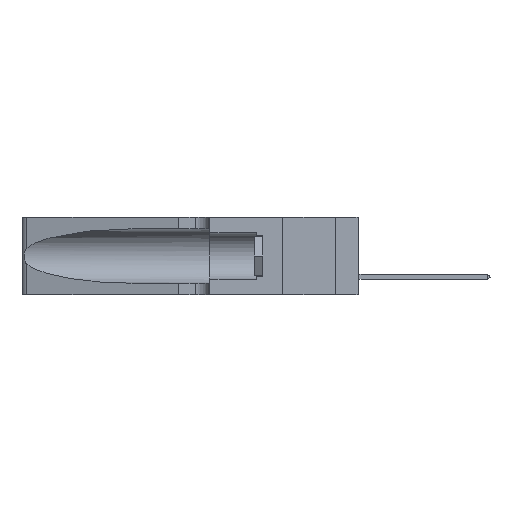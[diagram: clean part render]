
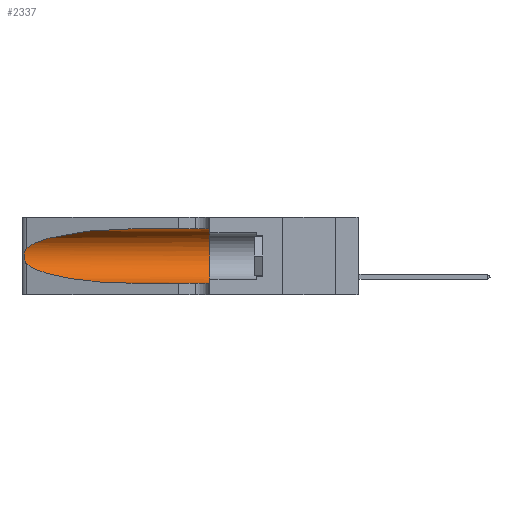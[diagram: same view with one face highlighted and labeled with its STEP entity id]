
A CAD part, left-side view. The second image highlights one B-rep face of the part: STEP entity #2337.
In plain terms, the highlighted cylindrical face has radius 3.308 mm (diameter 6.617 mm), a partial arc.
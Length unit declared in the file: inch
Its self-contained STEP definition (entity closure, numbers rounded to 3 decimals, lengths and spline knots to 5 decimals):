
#454 = CARTESIAN_POINT ( 'NONE',  ( 0.26075, 1.23896, 0.178 ) ) ;
#2295 = CARTESIAN_POINT ( 'NONE',  ( 0.25854, 1.2359, 0.20912 ) ) ;
#2337 = ADVANCED_FACE ( 'NONE', ( #6462 ), #10095, .F. ) ;
#2697 = EDGE_CURVE ( 'NONE', #14906, #32252, #18087, .T. ) ;
#2852 = VERTEX_POINT ( 'NONE', #28870 ) ;
#3932 = CARTESIAN_POINT ( 'NONE',  ( 0.1305, 0.72297, 0.31525 ) ) ;
#4654 = ORIENTED_EDGE ( 'NONE', *, *, #2697, .F. ) ;
#5775 = EDGE_CURVE ( 'NONE', #32252, #12425, #25843, .T. ) ;
#6020 = CARTESIAN_POINT ( 'NONE',  ( 0.2373, 1.15595, 0.08982 ) ) ;
#6446 = VERTEX_POINT ( 'NONE', #31807 ) ;
#6462 = FACE_OUTER_BOUND ( 'NONE', #29923, .T. ) ;
#6856 = VECTOR ( 'NONE', #22949, 39.37008 ) ;
#7241 = CARTESIAN_POINT ( 'NONE',  ( 0.25487, 1.22718, 0.22369 ) ) ;
#7370 = CARTESIAN_POINT ( 'NONE',  ( 0.25856, 1.23593, 0.16098 ) ) ;
#7404 = EDGE_CURVE ( 'NONE', #2852, #6446, #10278, .T. ) ;
#7745 = CARTESIAN_POINT ( 'NONE',  ( 0.1305, 1.61858, 0.31525 ) ) ;
#9529 = CARTESIAN_POINT ( 'NONE',  ( 0.1305, 0.72297, 0.05475 ) ) ;
#10095 = CYLINDRICAL_SURFACE ( 'NONE', #30429, 0.13025 ) ;
#10278 =( BOUNDED_CURVE ( )  B_SPLINE_CURVE ( 3, ( #33264, #6020, #31764, #9529 ),
 .UNSPECIFIED., .F., .T. ) 
 B_SPLINE_CURVE_WITH_KNOTS ( ( 4, 4 ),
 ( 3.44316, 4.71239 ),
 .UNSPECIFIED. ) 
 CURVE ( )  GEOMETRIC_REPRESENTATION_ITEM ( )  RATIONAL_B_SPLINE_CURVE ( ( 1., 0.87, 0.87, 1. ) ) 
 REPRESENTATION_ITEM ( '' )  );
#10597 = CARTESIAN_POINT ( 'NONE',  ( 0.26075, 1.23896, 0.19203 ) ) ;
#11135 = CARTESIAN_POINT ( 'NONE',  ( 0.1305, 1.61858, 0.185 ) ) ;
#11465 = DIRECTION ( 'NONE',  ( 0., 0., -1. ) ) ;
#11824 = DIRECTION ( 'NONE',  ( 0., 1., 0. ) ) ;
#12232 = CARTESIAN_POINT ( 'NONE',  ( 0.18966, 0.96281, 0.31525 ) ) ;
#12425 = VERTEX_POINT ( 'NONE', #19423 ) ;
#13458 = CARTESIAN_POINT ( 'NONE',  ( 0.1305, 1.61858, 0.05475 ) ) ;
#14906 = VERTEX_POINT ( 'NONE', #3932 ) ;
#15258 = CARTESIAN_POINT ( 'NONE',  ( 0.26018, 1.23835, 0.19895 ) ) ;
#15892 = CARTESIAN_POINT ( 'NONE',  ( 0.25789, 1.23486, 0.15765 ) ) ;
#15894 = EDGE_CURVE ( 'NONE', #6446, #12425, #19828, .T. ) ;
#17557 = AXIS2_PLACEMENT_3D ( 'NONE', #27231, #11824, #27682 ) ;
#17828 = CARTESIAN_POINT ( 'NONE',  ( 0.25555, 1.22993, 0.14849 ) ) ;
#18087 = LINE ( 'NONE', #7745, #6856 ) ;
#18279 =( BOUNDED_CURVE ( )  B_SPLINE_CURVE ( 3, ( #32993, #12232, #25368, #7241 ),
 .UNSPECIFIED., .F., .T. ) 
 B_SPLINE_CURVE_WITH_KNOTS ( ( 4, 4 ),
 ( 1.5708, 2.84003 ),
 .UNSPECIFIED. ) 
 CURVE ( )  GEOMETRIC_REPRESENTATION_ITEM ( )  RATIONAL_B_SPLINE_CURVE ( ( 1., 0.87, 0.87, 1. ) ) 
 REPRESENTATION_ITEM ( '' )  );
#18993 = VECTOR ( 'NONE', #31418, 39.37008 ) ;
#19423 = CARTESIAN_POINT ( 'NONE',  ( 0.1305, 0.35, 0.05475 ) ) ;
#19443 = ORIENTED_EDGE ( 'NONE', *, *, #5775, .F. ) ;
#19828 = LINE ( 'NONE', #13458, #18993 ) ;
#20319 = CARTESIAN_POINT ( 'NONE',  ( 0.25787, 1.23484, 0.2124 ) ) ;
#20538 = ORIENTED_EDGE ( 'NONE', *, *, #15894, .T. ) ;
#21029 = EDGE_CURVE ( 'NONE', #27607, #2852, #32774, .T. ) ;
#22562 = ORIENTED_EDGE ( 'NONE', *, *, #7404, .T. ) ;
#22949 = DIRECTION ( 'NONE',  ( 0., -1., 0. ) ) ;
#22960 = EDGE_CURVE ( 'NONE', #14906, #27607, #18279, .T. ) ;
#23156 = ORIENTED_EDGE ( 'NONE', *, *, #21029, .T. ) ;
#25368 = CARTESIAN_POINT ( 'NONE',  ( 0.2373, 1.15595, 0.28018 ) ) ;
#25386 = CARTESIAN_POINT ( 'NONE',  ( 0.25639, 1.23186, 0.15144 ) ) ;
#25495 = CARTESIAN_POINT ( 'NONE',  ( 0.25487, 1.22718, 0.22369 ) ) ;
#25510 = CARTESIAN_POINT ( 'NONE',  ( 0.25487, 1.22718, 0.22369 ) ) ;
#25843 = CIRCLE ( 'NONE', #17557, 0.13025 ) ;
#26920 = CARTESIAN_POINT ( 'NONE',  ( 0.1305, 0.35, 0.31525 ) ) ;
#27231 = CARTESIAN_POINT ( 'NONE',  ( 0.1305, 0.35, 0.185 ) ) ;
#27607 = VERTEX_POINT ( 'NONE', #25510 ) ;
#27682 = DIRECTION ( 'NONE',  ( 0., 0., 1. ) ) ;
#27969 = CARTESIAN_POINT ( 'NONE',  ( 0.26017, 1.23833, 0.17102 ) ) ;
#28849 = CARTESIAN_POINT ( 'NONE',  ( 0.25487, 1.22718, 0.14631 ) ) ;
#28870 = CARTESIAN_POINT ( 'NONE',  ( 0.25487, 1.22718, 0.14631 ) ) ;
#29145 = DIRECTION ( 'NONE',  ( 0., -1., 0. ) ) ;
#29923 = EDGE_LOOP ( 'NONE', ( #32422, #23156, #22562, #20538, #19443, #4654 ) ) ;
#30429 = AXIS2_PLACEMENT_3D ( 'NONE', #11135, #29145, #11465 ) ;
#30646 = CARTESIAN_POINT ( 'NONE',  ( 0.25639, 1.23184, 0.21858 ) ) ;
#31418 = DIRECTION ( 'NONE',  ( 0., -1., 0. ) ) ;
#31764 = CARTESIAN_POINT ( 'NONE',  ( 0.18966, 0.96281, 0.05475 ) ) ;
#31807 = CARTESIAN_POINT ( 'NONE',  ( 0.1305, 0.72297, 0.05475 ) ) ;
#32252 = VERTEX_POINT ( 'NONE', #26920 ) ;
#32422 = ORIENTED_EDGE ( 'NONE', *, *, #22960, .T. ) ;
#32774 = B_SPLINE_CURVE_WITH_KNOTS ( 'NONE', 3,
 ( #25495, #33122, #30646, #20319, #2295, #15258, #10597, #454, #27969, #7370, #15892, #25386, #17828, #28849 ),
 .UNSPECIFIED., .F., .F.,
 ( 4, 2, 2, 2, 2, 2, 4 ),
 ( 0., 0.00027, 0.00053, 0.00107, 0.0016, 0.00187, 0.00214 ),
 .UNSPECIFIED. ) ;
#32993 = CARTESIAN_POINT ( 'NONE',  ( 0.1305, 0.72297, 0.31525 ) ) ;
#33122 = CARTESIAN_POINT ( 'NONE',  ( 0.25555, 1.22994, 0.2215 ) ) ;
#33264 = CARTESIAN_POINT ( 'NONE',  ( 0.25487, 1.22718, 0.14631 ) ) ;
